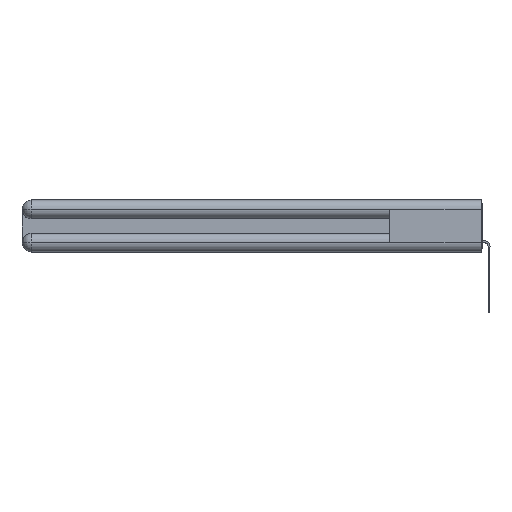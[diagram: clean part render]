
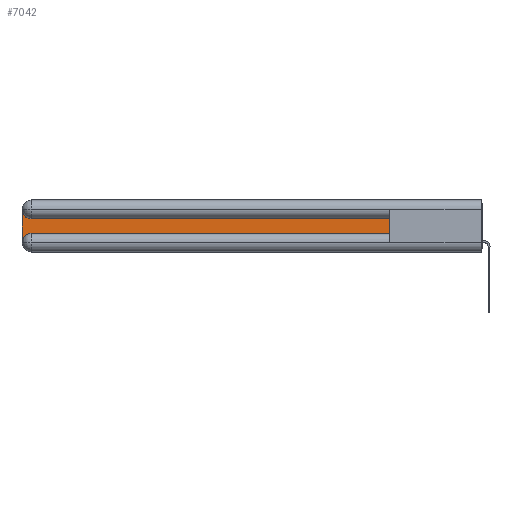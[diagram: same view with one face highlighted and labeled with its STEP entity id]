
A CAD part, left-side view. The second image highlights one B-rep face of the part: STEP entity #7042.
In plain terms, the highlighted planar face has unit normal (-1, 0, 0).
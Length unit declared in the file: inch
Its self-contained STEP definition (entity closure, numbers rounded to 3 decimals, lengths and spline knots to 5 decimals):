
#704 = AXIS2_PLACEMENT_3D ( 'NONE', #11373, #25611, #1315 ) ;
#1172 = ORIENTED_EDGE ( 'NONE', *, *, #6296, .T. ) ;
#1315 = DIRECTION ( 'NONE',  ( 0., 0., -1. ) ) ;
#2496 = EDGE_CURVE ( 'NONE', #5284, #22783, #2521, .T. ) ;
#2521 = LINE ( 'NONE', #10956, #20286 ) ;
#2595 = ORIENTED_EDGE ( 'NONE', *, *, #6208, .T. ) ;
#3723 = CARTESIAN_POINT ( 'NONE',  ( 0.075, 0.6, -0.1225 ) ) ;
#5038 = CARTESIAN_POINT ( 'NONE',  ( 0.075, 3., -0.2175 ) ) ;
#5202 = DIRECTION ( 'NONE',  ( 0., -1., 0. ) ) ;
#5284 = VERTEX_POINT ( 'NONE', #23298 ) ;
#5636 = VERTEX_POINT ( 'NONE', #3723 ) ;
#6208 = EDGE_CURVE ( 'NONE', #7807, #5284, #13684, .T. ) ;
#6296 = EDGE_CURVE ( 'NONE', #5636, #10223, #13069, .T. ) ;
#6568 = PLANE ( 'NONE',  #8291 ) ;
#7042 = ADVANCED_FACE ( 'NONE', ( #13958 ), #6568, .F. ) ;
#7807 = VERTEX_POINT ( 'NONE', #15613 ) ;
#8278 = DIRECTION ( 'NONE',  ( 1., 0., 0. ) ) ;
#8291 = AXIS2_PLACEMENT_3D ( 'NONE', #10628, #18814, #8764 ) ;
#8764 = DIRECTION ( 'NONE',  ( 0., 0., -1. ) ) ;
#9659 = VECTOR ( 'NONE', #25617, 39.37008 ) ;
#10223 = VERTEX_POINT ( 'NONE', #23467 ) ;
#10581 = CARTESIAN_POINT ( 'NONE',  ( 0.075, 3., -0.0625 ) ) ;
#10628 = CARTESIAN_POINT ( 'NONE',  ( 0.075, 3., -0.1225 ) ) ;
#10956 = CARTESIAN_POINT ( 'NONE',  ( 0.075, 0.6, -0.2175 ) ) ;
#11373 = CARTESIAN_POINT ( 'NONE',  ( 0.075, 2.94, -0.0625 ) ) ;
#11748 = EDGE_LOOP ( 'NONE', ( #1172, #21060, #15408, #2595, #21564, #21797 ) ) ;
#11982 = CARTESIAN_POINT ( 'NONE',  ( 0.075, 2.94, -0.2775 ) ) ;
#13069 = LINE ( 'NONE', #14297, #14662 ) ;
#13684 = CIRCLE ( 'NONE', #17969, 0.06 ) ;
#13757 = LINE ( 'NONE', #19408, #9659 ) ;
#13958 = FACE_OUTER_BOUND ( 'NONE', #11748, .T. ) ;
#14045 = CARTESIAN_POINT ( 'NONE',  ( 0.075, 0.6, -0.2175 ) ) ;
#14297 = CARTESIAN_POINT ( 'NONE',  ( 0.075, 0.6, -0.1225 ) ) ;
#14662 = VECTOR ( 'NONE', #24204, 39.37008 ) ;
#15133 = VERTEX_POINT ( 'NONE', #10581 ) ;
#15408 = ORIENTED_EDGE ( 'NONE', *, *, #18027, .T. ) ;
#15613 = CARTESIAN_POINT ( 'NONE',  ( 0.075, 3., -0.2775 ) ) ;
#17969 = AXIS2_PLACEMENT_3D ( 'NONE', #11982, #8278, #22437 ) ;
#18027 = EDGE_CURVE ( 'NONE', #15133, #7807, #25325, .T. ) ;
#18779 = EDGE_CURVE ( 'NONE', #10223, #15133, #19600, .T. ) ;
#18814 = DIRECTION ( 'NONE',  ( 1., 0., 0. ) ) ;
#19408 = CARTESIAN_POINT ( 'NONE',  ( 0.075, 0.6, -0.2175 ) ) ;
#19600 = CIRCLE ( 'NONE', #704, 0.06 ) ;
#20286 = VECTOR ( 'NONE', #5202, 39.37008 ) ;
#21060 = ORIENTED_EDGE ( 'NONE', *, *, #18779, .T. ) ;
#21564 = ORIENTED_EDGE ( 'NONE', *, *, #2496, .T. ) ;
#21565 = DIRECTION ( 'NONE',  ( 0., 0., -1. ) ) ;
#21797 = ORIENTED_EDGE ( 'NONE', *, *, #21820, .T. ) ;
#21820 = EDGE_CURVE ( 'NONE', #22783, #5636, #13757, .T. ) ;
#22437 = DIRECTION ( 'NONE',  ( 0., 0., -1. ) ) ;
#22783 = VERTEX_POINT ( 'NONE', #14045 ) ;
#23298 = CARTESIAN_POINT ( 'NONE',  ( 0.075, 2.94, -0.2175 ) ) ;
#23467 = CARTESIAN_POINT ( 'NONE',  ( 0.075, 2.94, -0.1225 ) ) ;
#24204 = DIRECTION ( 'NONE',  ( 0., 1., 0. ) ) ;
#24687 = VECTOR ( 'NONE', #21565, 39.37008 ) ;
#25325 = LINE ( 'NONE', #5038, #24687 ) ;
#25611 = DIRECTION ( 'NONE',  ( 1., 0., 0. ) ) ;
#25617 = DIRECTION ( 'NONE',  ( 0., 0., 1. ) ) ;
